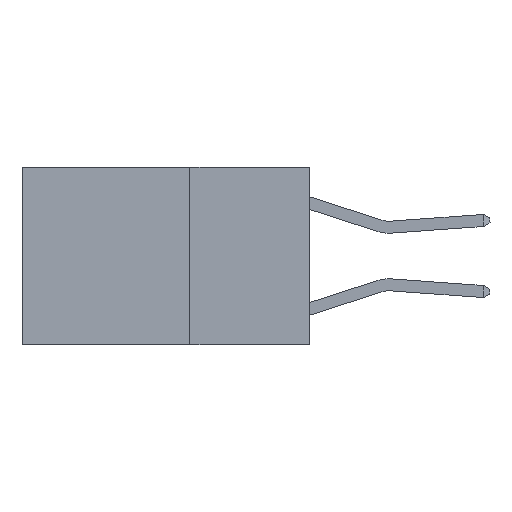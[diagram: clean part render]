
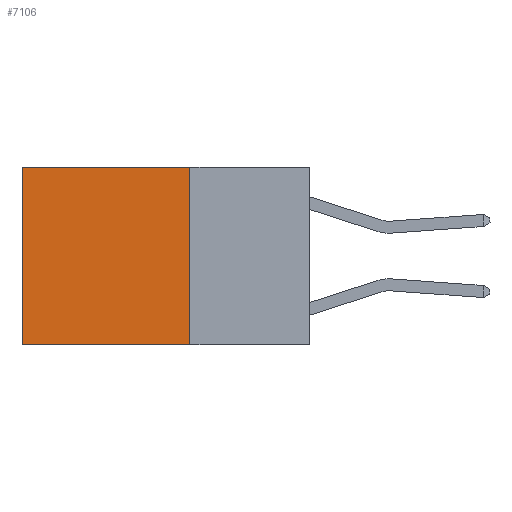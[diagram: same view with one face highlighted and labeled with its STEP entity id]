
A CAD part, left-side view. The second image highlights one B-rep face of the part: STEP entity #7106.
In plain terms, the highlighted planar face has unit normal (-1, 0, 0).
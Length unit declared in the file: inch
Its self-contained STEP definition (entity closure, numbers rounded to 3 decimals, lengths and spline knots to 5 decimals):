
#1640 = LINE ( 'NONE', #2782, #17850 ) ;
#1737 = ORIENTED_EDGE ( 'NONE', *, *, #21033, .T. ) ;
#1916 = DIRECTION ( 'NONE',  ( 0., 1., 0. ) ) ;
#2072 = DIRECTION ( 'NONE',  ( 1., 0., 0. ) ) ;
#2462 = VECTOR ( 'NONE', #23880, 39.37008 ) ;
#2699 = CARTESIAN_POINT ( 'NONE',  ( 0.2625, 0.6, -0.37 ) ) ;
#2782 = CARTESIAN_POINT ( 'NONE',  ( 0.2625, 0.25, 0. ) ) ;
#3161 = LINE ( 'NONE', #21629, #2462 ) ;
#3317 = EDGE_CURVE ( 'NONE', #12327, #12964, #13876, .T. ) ;
#3794 = ORIENTED_EDGE ( 'NONE', *, *, #18156, .F. ) ;
#3900 = VECTOR ( 'NONE', #1916, 39.37008 ) ;
#5046 = AXIS2_PLACEMENT_3D ( 'NONE', #13088, #2072, #17497 ) ;
#5106 = CARTESIAN_POINT ( 'NONE',  ( 0.2625, 0.6, 0. ) ) ;
#6102 = VERTEX_POINT ( 'NONE', #22827 ) ;
#6473 = FACE_OUTER_BOUND ( 'NONE', #21769, .T. ) ;
#7106 = ADVANCED_FACE ( 'NONE', ( #6473 ), #26287, .F. ) ;
#8748 = VECTOR ( 'NONE', #21518, 39.37008 ) ;
#12327 = VERTEX_POINT ( 'NONE', #5106 ) ;
#12964 = VERTEX_POINT ( 'NONE', #2699 ) ;
#13088 = CARTESIAN_POINT ( 'NONE',  ( 0.2625, 0.25, 0. ) ) ;
#13271 = ORIENTED_EDGE ( 'NONE', *, *, #3317, .T. ) ;
#13876 = LINE ( 'NONE', #19296, #8748 ) ;
#17497 = DIRECTION ( 'NONE',  ( 0., 0., -1. ) ) ;
#17850 = VECTOR ( 'NONE', #22619, 39.37008 ) ;
#18156 = EDGE_CURVE ( 'NONE', #6102, #12964, #21452, .T. ) ;
#18706 = EDGE_CURVE ( 'NONE', #26602, #6102, #3161, .T. ) ;
#19033 = CARTESIAN_POINT ( 'NONE',  ( 0.2625, 0.25, 0. ) ) ;
#19296 = CARTESIAN_POINT ( 'NONE',  ( 0.2625, 0.6, 0. ) ) ;
#21033 = EDGE_CURVE ( 'NONE', #26602, #12327, #1640, .T. ) ;
#21452 = LINE ( 'NONE', #28323, #3900 ) ;
#21518 = DIRECTION ( 'NONE',  ( 0., 0., -1. ) ) ;
#21629 = CARTESIAN_POINT ( 'NONE',  ( 0.2625, 0.25, 0. ) ) ;
#21769 = EDGE_LOOP ( 'NONE', ( #13271, #3794, #27573, #1737 ) ) ;
#22619 = DIRECTION ( 'NONE',  ( 0., 1., 0. ) ) ;
#22827 = CARTESIAN_POINT ( 'NONE',  ( 0.2625, 0.25, -0.37 ) ) ;
#23880 = DIRECTION ( 'NONE',  ( 0., 0., -1. ) ) ;
#26287 = PLANE ( 'NONE',  #5046 ) ;
#26602 = VERTEX_POINT ( 'NONE', #19033 ) ;
#27573 = ORIENTED_EDGE ( 'NONE', *, *, #18706, .F. ) ;
#28323 = CARTESIAN_POINT ( 'NONE',  ( 0.2625, 0.25, -0.37 ) ) ;
